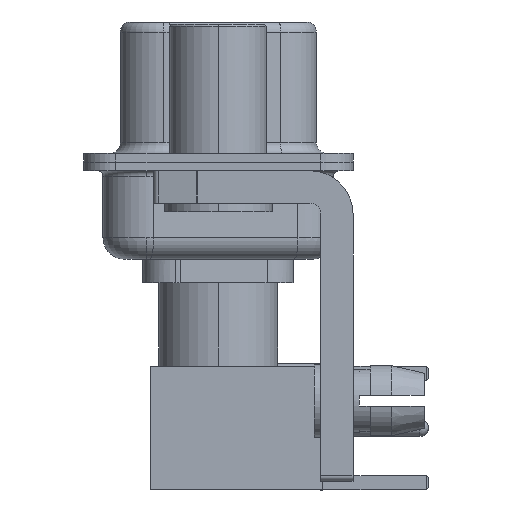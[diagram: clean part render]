
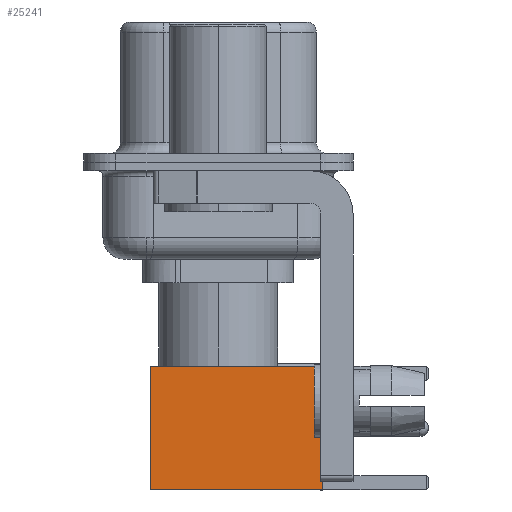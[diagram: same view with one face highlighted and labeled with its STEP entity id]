
A CAD part, left-side view. The second image highlights one B-rep face of the part: STEP entity #25241.
In plain terms, the highlighted face is planar.
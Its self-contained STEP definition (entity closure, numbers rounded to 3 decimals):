
#1259 = CARTESIAN_POINT ( 'NONE',  ( -2.875, 2.875, 8. ) ) ;
#1507 = LINE ( 'NONE', #32904, #20820 ) ;
#1666 = PLANE ( 'NONE',  #28060 ) ;
#2028 = LINE ( 'NONE', #16593, #27516 ) ;
#2249 = CARTESIAN_POINT ( 'NONE',  ( 2.875, 2.875, 8. ) ) ;
#2327 = EDGE_CURVE ( 'NONE', #25479, #16107, #2028, .T. ) ;
#3531 = CARTESIAN_POINT ( 'NONE',  ( -2.875, 2.875, 0. ) ) ;
#6197 = VECTOR ( 'NONE', #27526, 1000. ) ;
#7023 = LINE ( 'NONE', #35075, #28515 ) ;
#7519 = CARTESIAN_POINT ( 'NONE',  ( 2.875, 2.875, 0. ) ) ;
#8036 = CARTESIAN_POINT ( 'NONE',  ( 2.875, 2.875, 0. ) ) ;
#10555 = EDGE_CURVE ( 'NONE', #33649, #16107, #7023, .T. ) ;
#12924 = LINE ( 'NONE', #7519, #6197 ) ;
#13403 = EDGE_CURVE ( 'NONE', #27739, #25479, #1507, .T. ) ;
#14155 = EDGE_LOOP ( 'NONE', ( #29938, #35752, #31911, #23579 ) ) ;
#15258 = DIRECTION ( 'NONE',  ( -1., 0., 0. ) ) ;
#15880 = FACE_OUTER_BOUND ( 'NONE', #14155, .T. ) ;
#16107 = VERTEX_POINT ( 'NONE', #3531 ) ;
#16593 = CARTESIAN_POINT ( 'NONE',  ( -2.875, 2.875, 0. ) ) ;
#19429 = DIRECTION ( 'NONE',  ( 0., 1., 0. ) ) ;
#20820 = VECTOR ( 'NONE', #36093, 1000. ) ;
#23579 = ORIENTED_EDGE ( 'NONE', *, *, #13403, .F. ) ;
#25241 = ADVANCED_FACE ( 'NONE', ( #15880 ), #1666, .T. ) ;
#25479 = VERTEX_POINT ( 'NONE', #1259 ) ;
#27516 = VECTOR ( 'NONE', #31158, 1000. ) ;
#27526 = DIRECTION ( 'NONE',  ( 0., 0., -1. ) ) ;
#27739 = VERTEX_POINT ( 'NONE', #2249 ) ;
#28060 = AXIS2_PLACEMENT_3D ( 'NONE', #8036, #19429, #30806 ) ;
#28515 = VECTOR ( 'NONE', #15258, 1000. ) ;
#29266 = CARTESIAN_POINT ( 'NONE',  ( 2.875, 2.875, 0. ) ) ;
#29938 = ORIENTED_EDGE ( 'NONE', *, *, #34214, .T. ) ;
#30806 = DIRECTION ( 'NONE',  ( 0., 0., 1. ) ) ;
#31158 = DIRECTION ( 'NONE',  ( 0., 0., -1. ) ) ;
#31911 = ORIENTED_EDGE ( 'NONE', *, *, #2327, .F. ) ;
#32904 = CARTESIAN_POINT ( 'NONE',  ( 0., 2.875, 8. ) ) ;
#33649 = VERTEX_POINT ( 'NONE', #29266 ) ;
#34214 = EDGE_CURVE ( 'NONE', #27739, #33649, #12924, .T. ) ;
#35075 = CARTESIAN_POINT ( 'NONE',  ( 0., 2.875, 0. ) ) ;
#35752 = ORIENTED_EDGE ( 'NONE', *, *, #10555, .T. ) ;
#36093 = DIRECTION ( 'NONE',  ( -1., 0., 0. ) ) ;
